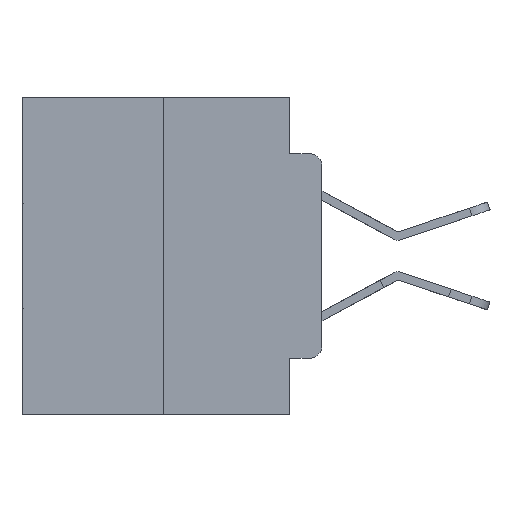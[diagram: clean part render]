
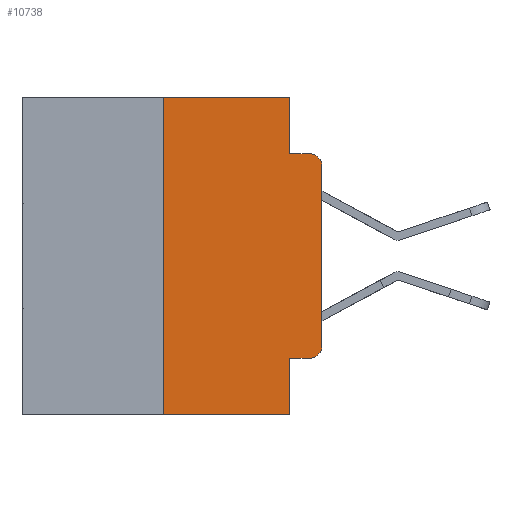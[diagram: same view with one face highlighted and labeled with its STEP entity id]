
A CAD part, left-side view. The second image highlights one B-rep face of the part: STEP entity #10738.
In plain terms, the highlighted planar face has unit normal (-1, 0, 0).
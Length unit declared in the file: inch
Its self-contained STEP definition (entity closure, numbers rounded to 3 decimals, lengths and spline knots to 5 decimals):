
#839 = VERTEX_POINT ( 'NONE', #1470 ) ;
#981 = AXIS2_PLACEMENT_3D ( 'NONE', #10717, #25352, #12831 ) ;
#1470 = CARTESIAN_POINT ( 'NONE',  ( 0., 0.051, -0.4115 ) ) ;
#1929 = EDGE_CURVE ( 'NONE', #839, #24496, #16237, .T. ) ;
#1967 = DIRECTION ( 'NONE',  ( 0., -1., 0. ) ) ;
#2095 = LINE ( 'NONE', #9733, #6544 ) ;
#2458 = EDGE_CURVE ( 'NONE', #6692, #11625, #21152, .T. ) ;
#2796 = DIRECTION ( 'NONE',  ( 0., -1., 0. ) ) ;
#3137 = CARTESIAN_POINT ( 'NONE',  ( 0., 0.25, 0. ) ) ;
#3228 = EDGE_CURVE ( 'NONE', #8277, #8477, #19487, .T. ) ;
#3513 = EDGE_CURVE ( 'NONE', #11625, #19952, #23727, .T. ) ;
#3726 = CARTESIAN_POINT ( 'NONE',  ( 0., 0.02, -0.3915 ) ) ;
#4462 = CARTESIAN_POINT ( 'NONE',  ( 0., 0.473, 0. ) ) ;
#5407 = CIRCLE ( 'NONE', #981, 0.02 ) ;
#5881 = CARTESIAN_POINT ( 'NONE',  ( 0., 0., -0.1085 ) ) ;
#6364 = VERTEX_POINT ( 'NONE', #22608 ) ;
#6544 = VECTOR ( 'NONE', #20219, 39.37008 ) ;
#6578 = DIRECTION ( 'NONE',  ( 0., 0., -1. ) ) ;
#6692 = VERTEX_POINT ( 'NONE', #17778 ) ;
#8112 = DIRECTION ( 'NONE',  ( 0., 0., -1. ) ) ;
#8277 = VERTEX_POINT ( 'NONE', #23350 ) ;
#8477 = VERTEX_POINT ( 'NONE', #13548 ) ;
#8818 = DIRECTION ( 'NONE',  ( 1., 0., 0. ) ) ;
#9733 = CARTESIAN_POINT ( 'NONE',  ( 0., 0.473, 0. ) ) ;
#9748 = CARTESIAN_POINT ( 'NONE',  ( 0., 0.051, -0.0885 ) ) ;
#10210 = EDGE_LOOP ( 'NONE', ( #25072, #11012, #10348, #22165, #26036, #23146, #17284, #22817, #10690, #27341 ) ) ;
#10280 = CARTESIAN_POINT ( 'NONE',  ( 0., 0.051, 0. ) ) ;
#10348 = ORIENTED_EDGE ( 'NONE', *, *, #3228, .F. ) ;
#10629 = EDGE_CURVE ( 'NONE', #6364, #24496, #21141, .T. ) ;
#10690 = ORIENTED_EDGE ( 'NONE', *, *, #23664, .T. ) ;
#10717 = CARTESIAN_POINT ( 'NONE',  ( 0., 0.02, -0.1085 ) ) ;
#10738 = ADVANCED_FACE ( 'NONE', ( #10957 ), #23404, .F. ) ;
#10957 = FACE_OUTER_BOUND ( 'NONE', #10210, .T. ) ;
#11012 = ORIENTED_EDGE ( 'NONE', *, *, #19531, .T. ) ;
#11150 = EDGE_CURVE ( 'NONE', #20952, #17101, #2095, .T. ) ;
#11625 = VERTEX_POINT ( 'NONE', #19746 ) ;
#12831 = DIRECTION ( 'NONE',  ( 0., 0., -1. ) ) ;
#13174 = EDGE_CURVE ( 'NONE', #17101, #8277, #22940, .T. ) ;
#13227 = VECTOR ( 'NONE', #2796, 39.37008 ) ;
#13548 = CARTESIAN_POINT ( 'NONE',  ( 0., 0.02, -0.0885 ) ) ;
#13621 = DIRECTION ( 'NONE',  ( 0., 0., 1. ) ) ;
#15552 = VECTOR ( 'NONE', #21845, 39.37008 ) ;
#15710 = AXIS2_PLACEMENT_3D ( 'NONE', #3726, #17338, #6578 ) ;
#15948 = CARTESIAN_POINT ( 'NONE',  ( 0., 0., 0. ) ) ;
#16237 = LINE ( 'NONE', #18482, #15552 ) ;
#16885 = CARTESIAN_POINT ( 'NONE',  ( 0., 0.473, -0.5 ) ) ;
#17101 = VERTEX_POINT ( 'NONE', #23115 ) ;
#17284 = ORIENTED_EDGE ( 'NONE', *, *, #10629, .T. ) ;
#17338 = DIRECTION ( 'NONE',  ( -1., 0., 0. ) ) ;
#17407 = VECTOR ( 'NONE', #8112, 39.37008 ) ;
#17778 = CARTESIAN_POINT ( 'NONE',  ( 0., 0.02, -0.4115 ) ) ;
#17862 = CARTESIAN_POINT ( 'NONE',  ( 0., 0.051, -0.5 ) ) ;
#18215 = VECTOR ( 'NONE', #13621, 39.37008 ) ;
#18482 = CARTESIAN_POINT ( 'NONE',  ( 0., 0.051, 0. ) ) ;
#18971 = DIRECTION ( 'NONE',  ( 0., -1., 0. ) ) ;
#19487 = LINE ( 'NONE', #9748, #13227 ) ;
#19531 = EDGE_CURVE ( 'NONE', #19952, #8477, #5407, .T. ) ;
#19746 = CARTESIAN_POINT ( 'NONE',  ( 0., 0., -0.3915 ) ) ;
#19840 = VECTOR ( 'NONE', #18971, 39.37008 ) ;
#19952 = VERTEX_POINT ( 'NONE', #5881 ) ;
#20219 = DIRECTION ( 'NONE',  ( 0., -1., 0. ) ) ;
#20952 = VERTEX_POINT ( 'NONE', #3137 ) ;
#21084 = CARTESIAN_POINT ( 'NONE',  ( 0., 0.051, -0.4115 ) ) ;
#21141 = LINE ( 'NONE', #16885, #19840 ) ;
#21152 = CIRCLE ( 'NONE', #15710, 0.02 ) ;
#21383 = LINE ( 'NONE', #24900, #24958 ) ;
#21845 = DIRECTION ( 'NONE',  ( 0., 0., -1. ) ) ;
#22165 = ORIENTED_EDGE ( 'NONE', *, *, #13174, .F. ) ;
#22608 = CARTESIAN_POINT ( 'NONE',  ( 0., 0.25, -0.5 ) ) ;
#22817 = ORIENTED_EDGE ( 'NONE', *, *, #1929, .F. ) ;
#22940 = LINE ( 'NONE', #10280, #17407 ) ;
#23115 = CARTESIAN_POINT ( 'NONE',  ( 0., 0.051, 0. ) ) ;
#23146 = ORIENTED_EDGE ( 'NONE', *, *, #25374, .F. ) ;
#23350 = CARTESIAN_POINT ( 'NONE',  ( 0., 0.051, -0.0885 ) ) ;
#23404 = PLANE ( 'NONE',  #24209 ) ;
#23492 = DIRECTION ( 'NONE',  ( 0., 0., -1. ) ) ;
#23664 = EDGE_CURVE ( 'NONE', #839, #6692, #25058, .T. ) ;
#23727 = LINE ( 'NONE', #15948, #18215 ) ;
#24209 = AXIS2_PLACEMENT_3D ( 'NONE', #4462, #8818, #23492 ) ;
#24408 = VECTOR ( 'NONE', #1967, 39.37008 ) ;
#24496 = VERTEX_POINT ( 'NONE', #17862 ) ;
#24900 = CARTESIAN_POINT ( 'NONE',  ( 0., 0.25, 0. ) ) ;
#24958 = VECTOR ( 'NONE', #26962, 39.37008 ) ;
#25058 = LINE ( 'NONE', #21084, #24408 ) ;
#25072 = ORIENTED_EDGE ( 'NONE', *, *, #3513, .T. ) ;
#25352 = DIRECTION ( 'NONE',  ( -1., 0., 0. ) ) ;
#25374 = EDGE_CURVE ( 'NONE', #6364, #20952, #21383, .T. ) ;
#26036 = ORIENTED_EDGE ( 'NONE', *, *, #11150, .F. ) ;
#26962 = DIRECTION ( 'NONE',  ( 0., 0., 1. ) ) ;
#27341 = ORIENTED_EDGE ( 'NONE', *, *, #2458, .T. ) ;
